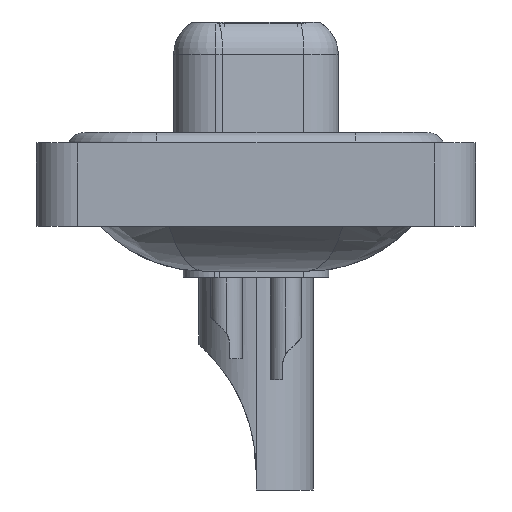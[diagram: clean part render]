
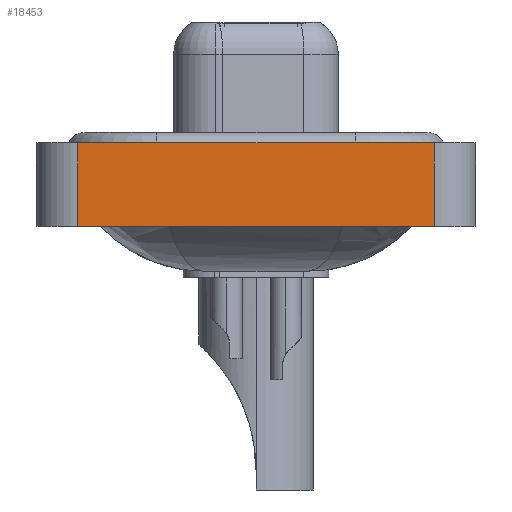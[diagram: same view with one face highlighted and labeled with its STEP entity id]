
A CAD part, left-side view. The second image highlights one B-rep face of the part: STEP entity #18453.
In plain terms, the highlighted planar face has unit normal (-1, 0, 0).
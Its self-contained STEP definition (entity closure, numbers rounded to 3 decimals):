
#427 = CARTESIAN_POINT ( 'NONE',  ( -7.35, -8.55, 0.4 ) ) ;
#736 = VECTOR ( 'NONE', #6915, 1000. ) ;
#4599 = LINE ( 'NONE', #25154, #22874 ) ;
#4953 = VERTEX_POINT ( 'NONE', #15669 ) ;
#5036 = VECTOR ( 'NONE', #8852, 1000. ) ;
#5093 = CARTESIAN_POINT ( 'NONE',  ( -7.35, -8.55, -3.6 ) ) ;
#5166 = VERTEX_POINT ( 'NONE', #23596 ) ;
#6915 = DIRECTION ( 'NONE',  ( 0., -1., 0. ) ) ;
#6962 = ORIENTED_EDGE ( 'NONE', *, *, #26277, .T. ) ;
#8245 = DIRECTION ( 'NONE',  ( 0., 0., 1. ) ) ;
#8323 = CARTESIAN_POINT ( 'NONE',  ( -7.35, -8.55, 0.4 ) ) ;
#8631 = DIRECTION ( 'NONE',  ( 0., 0., 1. ) ) ;
#8852 = DIRECTION ( 'NONE',  ( 0., 0., 1. ) ) ;
#8939 = LINE ( 'NONE', #13570, #736 ) ;
#9941 = LINE ( 'NONE', #8323, #25221 ) ;
#10293 = AXIS2_PLACEMENT_3D ( 'NONE', #16801, #24644, #8245 ) ;
#11392 = CARTESIAN_POINT ( 'NONE',  ( -7.35, -8.55, -3.6 ) ) ;
#12037 = EDGE_CURVE ( 'NONE', #4953, #19560, #9941, .T. ) ;
#13134 = LINE ( 'NONE', #5093, #5036 ) ;
#13162 = ORIENTED_EDGE ( 'NONE', *, *, #12037, .F. ) ;
#13570 = CARTESIAN_POINT ( 'NONE',  ( -7.35, -8.55, -3.6 ) ) ;
#13778 = ORIENTED_EDGE ( 'NONE', *, *, #16920, .F. ) ;
#15477 = ORIENTED_EDGE ( 'NONE', *, *, #17527, .T. ) ;
#15669 = CARTESIAN_POINT ( 'NONE',  ( -7.35, 8.55, 0.4 ) ) ;
#16082 = DIRECTION ( 'NONE',  ( 0., -1., 0. ) ) ;
#16204 = VERTEX_POINT ( 'NONE', #11392 ) ;
#16402 = FACE_OUTER_BOUND ( 'NONE', #21168, .T. ) ;
#16801 = CARTESIAN_POINT ( 'NONE',  ( -7.35, -8.55, -3.6 ) ) ;
#16920 = EDGE_CURVE ( 'NONE', #5166, #4953, #4599, .T. ) ;
#17527 = EDGE_CURVE ( 'NONE', #5166, #16204, #8939, .T. ) ;
#18453 = ADVANCED_FACE ( 'NONE', ( #16402 ), #22518, .T. ) ;
#19560 = VERTEX_POINT ( 'NONE', #427 ) ;
#21168 = EDGE_LOOP ( 'NONE', ( #6962, #13162, #13778, #15477 ) ) ;
#22518 = PLANE ( 'NONE',  #10293 ) ;
#22874 = VECTOR ( 'NONE', #8631, 1000. ) ;
#23596 = CARTESIAN_POINT ( 'NONE',  ( -7.35, 8.55, -3.6 ) ) ;
#24644 = DIRECTION ( 'NONE',  ( -1., 0., 0. ) ) ;
#25154 = CARTESIAN_POINT ( 'NONE',  ( -7.35, 8.55, -3.6 ) ) ;
#25221 = VECTOR ( 'NONE', #16082, 1000. ) ;
#26277 = EDGE_CURVE ( 'NONE', #16204, #19560, #13134, .T. ) ;
